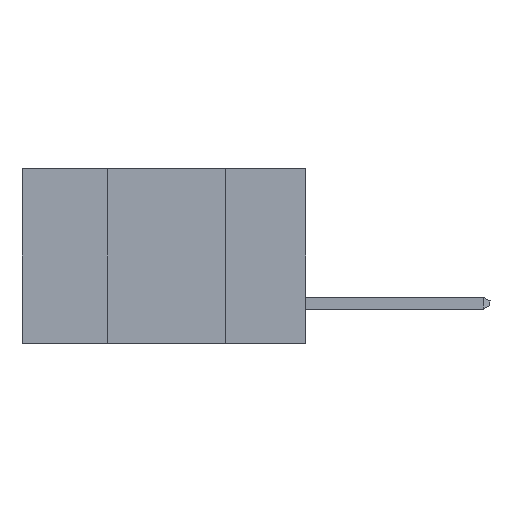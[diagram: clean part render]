
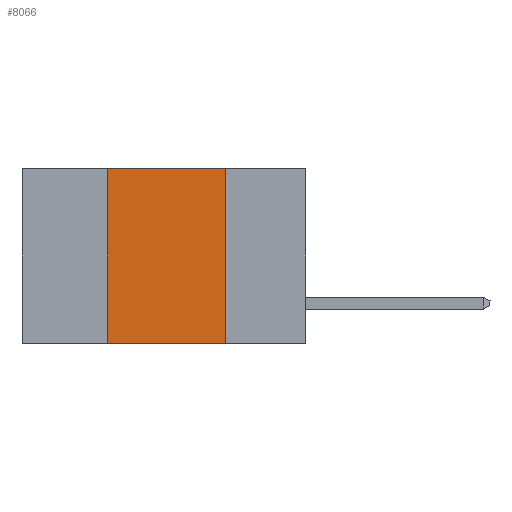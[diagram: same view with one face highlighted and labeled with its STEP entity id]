
A CAD part, left-side view. The second image highlights one B-rep face of the part: STEP entity #8066.
In plain terms, the highlighted planar face has unit normal (-1, 0, 0).
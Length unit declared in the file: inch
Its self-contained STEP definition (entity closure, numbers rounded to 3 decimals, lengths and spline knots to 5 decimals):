
#1660 = DIRECTION ( 'NONE',  ( 1., 0., 0. ) ) ;
#1693 = LINE ( 'NONE', #19051, #13001 ) ;
#2169 = LINE ( 'NONE', #7188, #9657 ) ;
#3304 = VECTOR ( 'NONE', #3786, 39.37008 ) ;
#3786 = DIRECTION ( 'NONE',  ( 0., -1., 0. ) ) ;
#3882 = ORIENTED_EDGE ( 'NONE', *, *, #5581, .F. ) ;
#4814 = EDGE_CURVE ( 'NONE', #11626, #14902, #2169, .T. ) ;
#5003 = CARTESIAN_POINT ( 'NONE',  ( 0., 0.17, 0. ) ) ;
#5581 = EDGE_CURVE ( 'NONE', #14902, #19753, #1693, .T. ) ;
#6008 = CARTESIAN_POINT ( 'NONE',  ( 0., 0.17, -0.37 ) ) ;
#7188 = CARTESIAN_POINT ( 'NONE',  ( 0., 0.42, -0.37 ) ) ;
#7407 = LINE ( 'NONE', #15277, #3304 ) ;
#7530 = DIRECTION ( 'NONE',  ( 0., 0., -1. ) ) ;
#8023 = ORIENTED_EDGE ( 'NONE', *, *, #4814, .F. ) ;
#8066 = ADVANCED_FACE ( 'NONE', ( #11346 ), #18075, .F. ) ;
#8178 = DIRECTION ( 'NONE',  ( 0., 0., -1. ) ) ;
#8381 = CARTESIAN_POINT ( 'NONE',  ( 0., 0.6, 0. ) ) ;
#8454 = EDGE_CURVE ( 'NONE', #19753, #11030, #14317, .T. ) ;
#8701 = CARTESIAN_POINT ( 'NONE',  ( 0., 0.42, -0.37 ) ) ;
#9391 = ORIENTED_EDGE ( 'NONE', *, *, #16676, .T. ) ;
#9657 = VECTOR ( 'NONE', #10056, 39.37008 ) ;
#10056 = DIRECTION ( 'NONE',  ( 0., 0., 1. ) ) ;
#10266 = VECTOR ( 'NONE', #7530, 39.37008 ) ;
#11030 = VERTEX_POINT ( 'NONE', #11700 ) ;
#11346 = FACE_OUTER_BOUND ( 'NONE', #15632, .T. ) ;
#11626 = VERTEX_POINT ( 'NONE', #8701 ) ;
#11700 = CARTESIAN_POINT ( 'NONE',  ( 0., 0.17, -0.37 ) ) ;
#13001 = VECTOR ( 'NONE', #19163, 39.37008 ) ;
#13072 = CARTESIAN_POINT ( 'NONE',  ( 0., 0.42, 0. ) ) ;
#14317 = LINE ( 'NONE', #6008, #10266 ) ;
#14902 = VERTEX_POINT ( 'NONE', #13072 ) ;
#15277 = CARTESIAN_POINT ( 'NONE',  ( 0., 0.6, -0.37 ) ) ;
#15632 = EDGE_LOOP ( 'NONE', ( #20083, #3882, #8023, #9391 ) ) ;
#16676 = EDGE_CURVE ( 'NONE', #11626, #11030, #7407, .T. ) ;
#17817 = AXIS2_PLACEMENT_3D ( 'NONE', #8381, #1660, #8178 ) ;
#18075 = PLANE ( 'NONE',  #17817 ) ;
#19051 = CARTESIAN_POINT ( 'NONE',  ( 0., 0.6, 0. ) ) ;
#19163 = DIRECTION ( 'NONE',  ( 0., -1., 0. ) ) ;
#19753 = VERTEX_POINT ( 'NONE', #5003 ) ;
#20083 = ORIENTED_EDGE ( 'NONE', *, *, #8454, .F. ) ;
